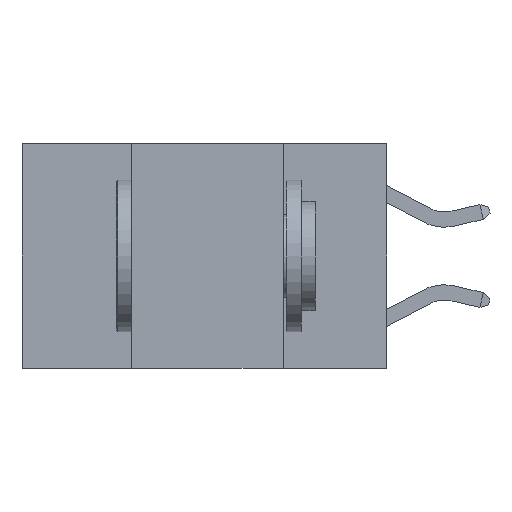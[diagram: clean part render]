
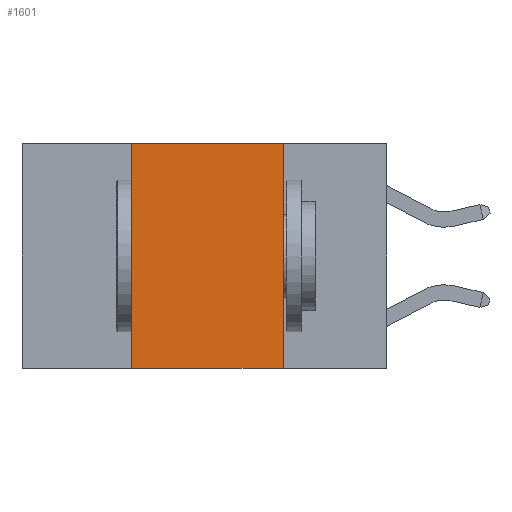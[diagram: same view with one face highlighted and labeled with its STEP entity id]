
A CAD part, left-side view. The second image highlights one B-rep face of the part: STEP entity #1601.
In plain terms, the highlighted planar face has unit normal (-1, 0, 0).
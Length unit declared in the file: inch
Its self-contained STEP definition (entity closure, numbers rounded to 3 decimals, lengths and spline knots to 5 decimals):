
#254 = CARTESIAN_POINT ( 'NONE',  ( 0., 0.6, 0. ) ) ;
#534 = CARTESIAN_POINT ( 'NONE',  ( 0., 0.42, -0.37 ) ) ;
#732 = DIRECTION ( 'NONE',  ( 0., -1., 0. ) ) ;
#1477 = CARTESIAN_POINT ( 'NONE',  ( 0., 0.17, -0.37 ) ) ;
#1601 = ADVANCED_FACE ( 'NONE', ( #2574 ), #3796, .F. ) ;
#2144 = EDGE_CURVE ( 'NONE', #9395, #4369, #9962, .T. ) ;
#2355 = VECTOR ( 'NONE', #3616, 39.37008 ) ;
#2574 = FACE_OUTER_BOUND ( 'NONE', #7016, .T. ) ;
#2938 = VECTOR ( 'NONE', #6333, 39.37008 ) ;
#2975 = VERTEX_POINT ( 'NONE', #1477 ) ;
#3296 = DIRECTION ( 'NONE',  ( 0., 0., -1. ) ) ;
#3434 = DIRECTION ( 'NONE',  ( 1., 0., 0. ) ) ;
#3482 = CARTESIAN_POINT ( 'NONE',  ( 0., 0.6, 0. ) ) ;
#3491 = CARTESIAN_POINT ( 'NONE',  ( 0., 0.17, 0. ) ) ;
#3616 = DIRECTION ( 'NONE',  ( 0., -1., 0. ) ) ;
#3636 = CARTESIAN_POINT ( 'NONE',  ( 0., 0.17, 0. ) ) ;
#3796 = PLANE ( 'NONE',  #4570 ) ;
#4369 = VERTEX_POINT ( 'NONE', #3636 ) ;
#4463 = ORIENTED_EDGE ( 'NONE', *, *, #11284, .F. ) ;
#4570 = AXIS2_PLACEMENT_3D ( 'NONE', #3482, #3434, #3296 ) ;
#4857 = LINE ( 'NONE', #7979, #2355 ) ;
#5471 = VECTOR ( 'NONE', #732, 39.37008 ) ;
#6333 = DIRECTION ( 'NONE',  ( 0., 0., 1. ) ) ;
#6936 = VERTEX_POINT ( 'NONE', #534 ) ;
#7016 = EDGE_LOOP ( 'NONE', ( #8776, #10962, #4463, #9046 ) ) ;
#7931 = EDGE_CURVE ( 'NONE', #6936, #2975, #4857, .T. ) ;
#7979 = CARTESIAN_POINT ( 'NONE',  ( 0., 0.6, -0.37 ) ) ;
#8238 = VECTOR ( 'NONE', #9582, 39.37008 ) ;
#8486 = LINE ( 'NONE', #3491, #8238 ) ;
#8776 = ORIENTED_EDGE ( 'NONE', *, *, #11203, .F. ) ;
#9046 = ORIENTED_EDGE ( 'NONE', *, *, #7931, .T. ) ;
#9395 = VERTEX_POINT ( 'NONE', #10200 ) ;
#9582 = DIRECTION ( 'NONE',  ( 0., 0., -1. ) ) ;
#9942 = LINE ( 'NONE', #11193, #2938 ) ;
#9962 = LINE ( 'NONE', #254, #5471 ) ;
#10200 = CARTESIAN_POINT ( 'NONE',  ( 0., 0.42, 0. ) ) ;
#10962 = ORIENTED_EDGE ( 'NONE', *, *, #2144, .F. ) ;
#11193 = CARTESIAN_POINT ( 'NONE',  ( 0., 0.42, 0. ) ) ;
#11203 = EDGE_CURVE ( 'NONE', #4369, #2975, #8486, .T. ) ;
#11284 = EDGE_CURVE ( 'NONE', #6936, #9395, #9942, .T. ) ;
